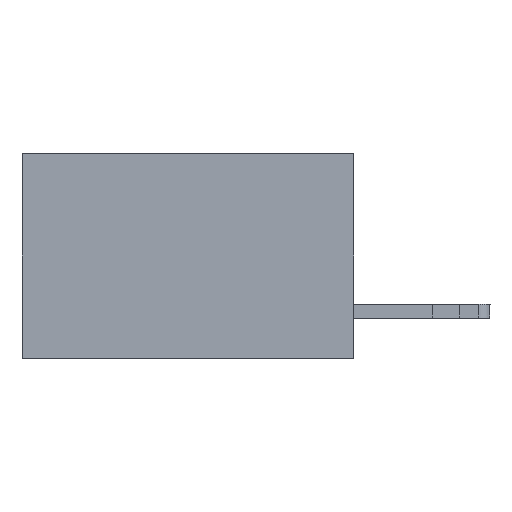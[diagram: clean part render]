
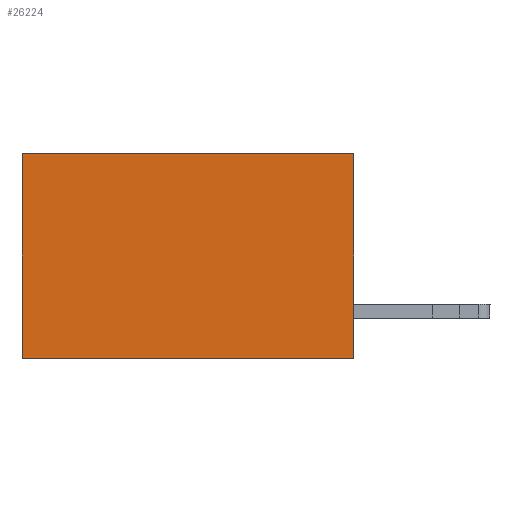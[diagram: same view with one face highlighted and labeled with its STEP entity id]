
A CAD part, left-side view. The second image highlights one B-rep face of the part: STEP entity #26224.
In plain terms, the highlighted planar face has unit normal (-1, 0, 0).
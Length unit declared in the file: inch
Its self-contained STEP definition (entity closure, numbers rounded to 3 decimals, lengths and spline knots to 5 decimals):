
#867 = VERTEX_POINT ( 'NONE', #7151 ) ;
#881 = ORIENTED_EDGE ( 'NONE', *, *, #12218, .T. ) ;
#2894 = LINE ( 'NONE', #22720, #3629 ) ;
#3373 = DIRECTION ( 'NONE',  ( 0., 1., 0. ) ) ;
#3629 = VECTOR ( 'NONE', #18212, 39.37008 ) ;
#5651 = VECTOR ( 'NONE', #7704, 39.37008 ) ;
#6794 = AXIS2_PLACEMENT_3D ( 'NONE', #18200, #24903, #11491 ) ;
#6998 = CARTESIAN_POINT ( 'NONE',  ( 0.2875, 0.6, 0. ) ) ;
#7151 = CARTESIAN_POINT ( 'NONE',  ( 0.2875, 0.6, -0.37 ) ) ;
#7557 = FACE_OUTER_BOUND ( 'NONE', #14686, .T. ) ;
#7704 = DIRECTION ( 'NONE',  ( 0., 0., -1. ) ) ;
#7899 = CARTESIAN_POINT ( 'NONE',  ( 0.2875, 0.6, 0. ) ) ;
#9758 = EDGE_CURVE ( 'NONE', #17109, #23884, #19053, .T. ) ;
#10263 = ORIENTED_EDGE ( 'NONE', *, *, #14322, .T. ) ;
#10417 = VECTOR ( 'NONE', #15877, 39.37008 ) ;
#11491 = DIRECTION ( 'NONE',  ( 0., 0., -1. ) ) ;
#11503 = LINE ( 'NONE', #6998, #10417 ) ;
#12018 = CARTESIAN_POINT ( 'NONE',  ( 0.2875, 0., -0.37 ) ) ;
#12218 = EDGE_CURVE ( 'NONE', #17055, #867, #11503, .T. ) ;
#12558 = VECTOR ( 'NONE', #3373, 39.37008 ) ;
#14322 = EDGE_CURVE ( 'NONE', #17109, #17055, #2894, .T. ) ;
#14686 = EDGE_LOOP ( 'NONE', ( #881, #18307, #24239, #10263 ) ) ;
#15877 = DIRECTION ( 'NONE',  ( 0., 0., -1. ) ) ;
#16342 = LINE ( 'NONE', #23488, #12558 ) ;
#17054 = CARTESIAN_POINT ( 'NONE',  ( 0.2875, 0., 0. ) ) ;
#17055 = VERTEX_POINT ( 'NONE', #7899 ) ;
#17109 = VERTEX_POINT ( 'NONE', #17054 ) ;
#17598 = EDGE_CURVE ( 'NONE', #23884, #867, #16342, .T. ) ;
#18200 = CARTESIAN_POINT ( 'NONE',  ( 0.2875, 0., 0. ) ) ;
#18212 = DIRECTION ( 'NONE',  ( 0., 1., 0. ) ) ;
#18307 = ORIENTED_EDGE ( 'NONE', *, *, #17598, .F. ) ;
#18479 = PLANE ( 'NONE',  #6794 ) ;
#19053 = LINE ( 'NONE', #20948, #5651 ) ;
#20948 = CARTESIAN_POINT ( 'NONE',  ( 0.2875, 0., 0. ) ) ;
#22720 = CARTESIAN_POINT ( 'NONE',  ( 0.2875, 0., 0. ) ) ;
#23488 = CARTESIAN_POINT ( 'NONE',  ( 0.2875, 0., -0.37 ) ) ;
#23884 = VERTEX_POINT ( 'NONE', #12018 ) ;
#24239 = ORIENTED_EDGE ( 'NONE', *, *, #9758, .F. ) ;
#24903 = DIRECTION ( 'NONE',  ( 1., 0., 0. ) ) ;
#26224 = ADVANCED_FACE ( 'NONE', ( #7557 ), #18479, .F. ) ;
